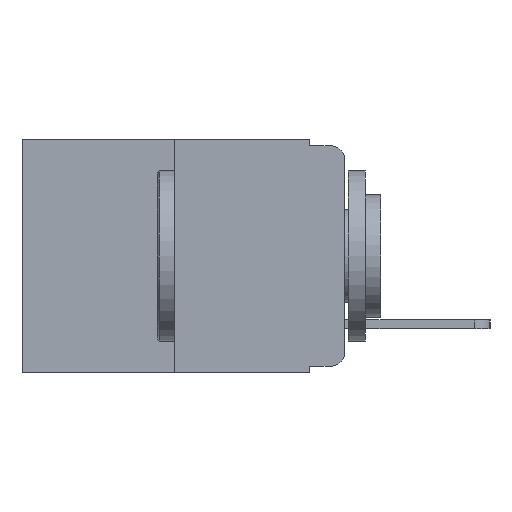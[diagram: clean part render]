
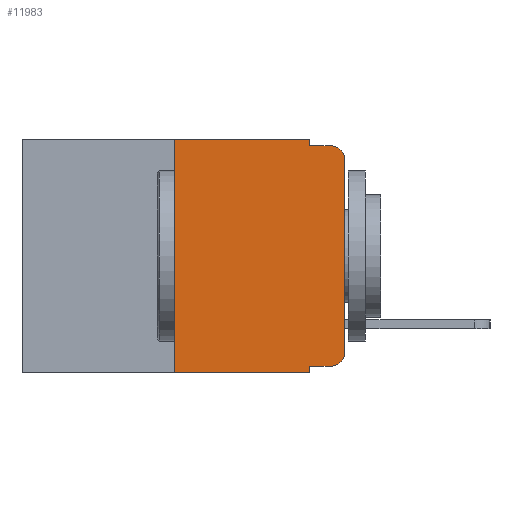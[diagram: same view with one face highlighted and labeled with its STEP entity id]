
A CAD part, left-side view. The second image highlights one B-rep face of the part: STEP entity #11983.
In plain terms, the highlighted planar face has unit normal (-1, 0, 0).
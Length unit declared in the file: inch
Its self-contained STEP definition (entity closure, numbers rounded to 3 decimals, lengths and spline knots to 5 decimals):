
#97 = VERTEX_POINT ( 'NONE', #9365 ) ;
#140 = CARTESIAN_POINT ( 'NONE',  ( 0., 0.051, -0.333 ) ) ;
#189 = CARTESIAN_POINT ( 'NONE',  ( 0., 0.051, -0.343 ) ) ;
#398 = CARTESIAN_POINT ( 'NONE',  ( 0., 0.02, -0.333 ) ) ;
#413 = VECTOR ( 'NONE', #14750, 39.37008 ) ;
#727 = CARTESIAN_POINT ( 'NONE',  ( 0., 0.051, 0. ) ) ;
#756 = CARTESIAN_POINT ( 'NONE',  ( 0., 0.25, 0. ) ) ;
#764 = CARTESIAN_POINT ( 'NONE',  ( 0., 0.473, 0. ) ) ;
#869 = VERTEX_POINT ( 'NONE', #15004 ) ;
#1168 = CIRCLE ( 'NONE', #1209, 0.02 ) ;
#1185 = VERTEX_POINT ( 'NONE', #8840 ) ;
#1209 = AXIS2_PLACEMENT_3D ( 'NONE', #16661, #8165, #18072 ) ;
#1711 = VERTEX_POINT ( 'NONE', #2728 ) ;
#2229 = ORIENTED_EDGE ( 'NONE', *, *, #17750, .F. ) ;
#2728 = CARTESIAN_POINT ( 'NONE',  ( 0., 0.25, -0.343 ) ) ;
#3451 = EDGE_CURVE ( 'NONE', #1185, #15041, #9404, .T. ) ;
#3759 = EDGE_CURVE ( 'NONE', #9831, #11804, #4646, .T. ) ;
#3841 = LINE ( 'NONE', #764, #6773 ) ;
#4451 = ORIENTED_EDGE ( 'NONE', *, *, #18462, .T. ) ;
#4646 = LINE ( 'NONE', #10515, #15172 ) ;
#4676 = EDGE_CURVE ( 'NONE', #97, #1185, #11379, .T. ) ;
#5079 = DIRECTION ( 'NONE',  ( 0., 0., 1. ) ) ;
#5097 = CARTESIAN_POINT ( 'NONE',  ( 0., 0.473, 0. ) ) ;
#5328 = VERTEX_POINT ( 'NONE', #14276 ) ;
#5359 = CARTESIAN_POINT ( 'NONE',  ( 0., 0., 0. ) ) ;
#5674 = DIRECTION ( 'NONE',  ( 0., 0., 1. ) ) ;
#5809 = EDGE_CURVE ( 'NONE', #1711, #11120, #7741, .T. ) ;
#6128 = LINE ( 'NONE', #756, #13739 ) ;
#6271 = VECTOR ( 'NONE', #15200, 39.37008 ) ;
#6542 = DIRECTION ( 'NONE',  ( 0., 0., -1. ) ) ;
#6773 = VECTOR ( 'NONE', #9408, 39.37008 ) ;
#6826 = VECTOR ( 'NONE', #18200, 39.37008 ) ;
#6937 = EDGE_CURVE ( 'NONE', #5328, #11346, #3841, .T. ) ;
#7172 = ORIENTED_EDGE ( 'NONE', *, *, #4676, .T. ) ;
#7741 = LINE ( 'NONE', #15385, #6826 ) ;
#7840 = LINE ( 'NONE', #16156, #15408 ) ;
#7866 = ORIENTED_EDGE ( 'NONE', *, *, #3759, .T. ) ;
#8165 = DIRECTION ( 'NONE',  ( -1., 0., 0. ) ) ;
#8674 = EDGE_CURVE ( 'NONE', #869, #15041, #14736, .T. ) ;
#8840 = CARTESIAN_POINT ( 'NONE',  ( 0., 0., -0.03 ) ) ;
#8989 = ORIENTED_EDGE ( 'NONE', *, *, #13901, .F. ) ;
#9365 = CARTESIAN_POINT ( 'NONE',  ( 0., 0., -0.313 ) ) ;
#9404 = CIRCLE ( 'NONE', #13623, 0.02 ) ;
#9408 = DIRECTION ( 'NONE',  ( 0., -1., 0. ) ) ;
#9831 = VERTEX_POINT ( 'NONE', #140 ) ;
#10515 = CARTESIAN_POINT ( 'NONE',  ( 0., 0.051, -0.333 ) ) ;
#10536 = DIRECTION ( 'NONE',  ( 0., 0., -1. ) ) ;
#11031 = DIRECTION ( 'NONE',  ( 0., 0., -1. ) ) ;
#11120 = VERTEX_POINT ( 'NONE', #189 ) ;
#11338 = EDGE_LOOP ( 'NONE', ( #7172, #11438, #12325, #8989, #16533, #2229, #14535, #14975, #7866, #4451 ) ) ;
#11346 = VERTEX_POINT ( 'NONE', #727 ) ;
#11379 = LINE ( 'NONE', #5359, #15127 ) ;
#11438 = ORIENTED_EDGE ( 'NONE', *, *, #3451, .T. ) ;
#11782 = CARTESIAN_POINT ( 'NONE',  ( 0., 0.02, -0.03 ) ) ;
#11804 = VERTEX_POINT ( 'NONE', #398 ) ;
#11955 = DIRECTION ( 'NONE',  ( -1., 0., 0. ) ) ;
#11983 = ADVANCED_FACE ( 'NONE', ( #14191 ), #13665, .F. ) ;
#12325 = ORIENTED_EDGE ( 'NONE', *, *, #8674, .F. ) ;
#13324 = CARTESIAN_POINT ( 'NONE',  ( 0., 0.051, -0.01 ) ) ;
#13623 = AXIS2_PLACEMENT_3D ( 'NONE', #11782, #11955, #11031 ) ;
#13665 = PLANE ( 'NONE',  #17242 ) ;
#13739 = VECTOR ( 'NONE', #5079, 39.37008 ) ;
#13761 = CARTESIAN_POINT ( 'NONE',  ( 0., 0.051, 0. ) ) ;
#13901 = EDGE_CURVE ( 'NONE', #11346, #869, #15221, .T. ) ;
#14191 = FACE_OUTER_BOUND ( 'NONE', #11338, .T. ) ;
#14276 = CARTESIAN_POINT ( 'NONE',  ( 0., 0.25, 0. ) ) ;
#14384 = DIRECTION ( 'NONE',  ( 0., -1., 0. ) ) ;
#14535 = ORIENTED_EDGE ( 'NONE', *, *, #5809, .T. ) ;
#14736 = LINE ( 'NONE', #13324, #413 ) ;
#14750 = DIRECTION ( 'NONE',  ( 0., -1., 0. ) ) ;
#14861 = EDGE_CURVE ( 'NONE', #9831, #11120, #7840, .T. ) ;
#14975 = ORIENTED_EDGE ( 'NONE', *, *, #14861, .F. ) ;
#15004 = CARTESIAN_POINT ( 'NONE',  ( 0., 0.051, -0.01 ) ) ;
#15032 = DIRECTION ( 'NONE',  ( 1., 0., 0. ) ) ;
#15041 = VERTEX_POINT ( 'NONE', #15093 ) ;
#15093 = CARTESIAN_POINT ( 'NONE',  ( 0., 0.02, -0.01 ) ) ;
#15127 = VECTOR ( 'NONE', #5674, 39.37008 ) ;
#15172 = VECTOR ( 'NONE', #14384, 39.37008 ) ;
#15200 = DIRECTION ( 'NONE',  ( 0., 0., -1. ) ) ;
#15221 = LINE ( 'NONE', #13761, #6271 ) ;
#15385 = CARTESIAN_POINT ( 'NONE',  ( 0., 0.473, -0.343 ) ) ;
#15408 = VECTOR ( 'NONE', #10536, 39.37008 ) ;
#16156 = CARTESIAN_POINT ( 'NONE',  ( 0., 0.051, 0. ) ) ;
#16533 = ORIENTED_EDGE ( 'NONE', *, *, #6937, .F. ) ;
#16661 = CARTESIAN_POINT ( 'NONE',  ( 0., 0.02, -0.313 ) ) ;
#17242 = AXIS2_PLACEMENT_3D ( 'NONE', #5097, #15032, #6542 ) ;
#17750 = EDGE_CURVE ( 'NONE', #1711, #5328, #6128, .T. ) ;
#18072 = DIRECTION ( 'NONE',  ( 0., 0., -1. ) ) ;
#18200 = DIRECTION ( 'NONE',  ( 0., -1., 0. ) ) ;
#18462 = EDGE_CURVE ( 'NONE', #11804, #97, #1168, .T. ) ;
